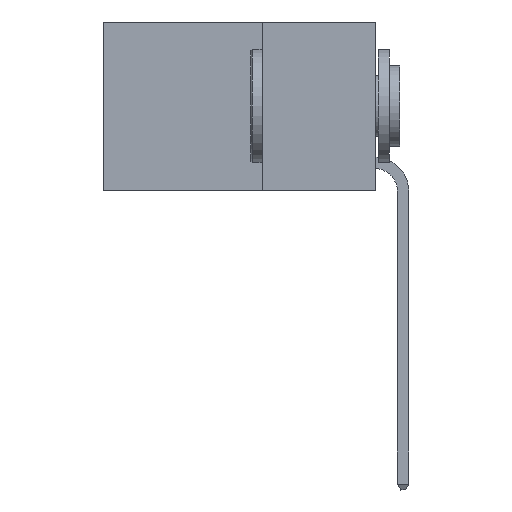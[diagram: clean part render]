
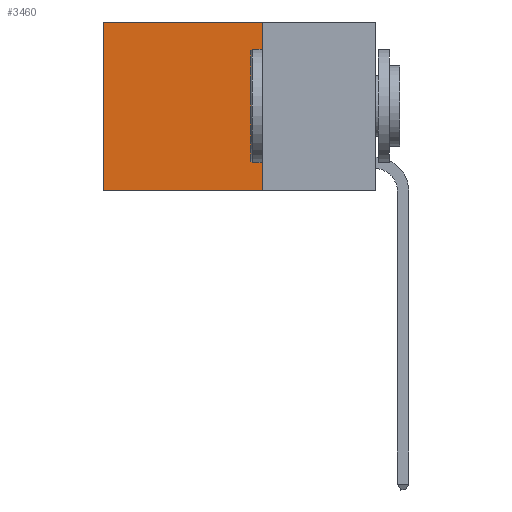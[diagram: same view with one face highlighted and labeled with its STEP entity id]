
A CAD part, left-side view. The second image highlights one B-rep face of the part: STEP entity #3460.
In plain terms, the highlighted planar face has unit normal (-1, 0, 0).
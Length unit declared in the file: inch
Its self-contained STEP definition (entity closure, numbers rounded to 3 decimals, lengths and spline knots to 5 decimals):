
#1109 = VERTEX_POINT ( 'NONE', #20126 ) ;
#1355 = ORIENTED_EDGE ( 'NONE', *, *, #22848, .T. ) ;
#1933 = CARTESIAN_POINT ( 'NONE',  ( 0.2625, 0.25, 0. ) ) ;
#2531 = DIRECTION ( 'NONE',  ( 1., 0., 0. ) ) ;
#3460 = ADVANCED_FACE ( 'NONE', ( #25578 ), #28165, .F. ) ;
#7009 = CARTESIAN_POINT ( 'NONE',  ( 0.2625, 0.6, 0. ) ) ;
#8017 = LINE ( 'NONE', #26478, #14754 ) ;
#8722 = EDGE_CURVE ( 'NONE', #28034, #11295, #30033, .T. ) ;
#8973 = DIRECTION ( 'NONE',  ( 0., 0., -1. ) ) ;
#8996 = CARTESIAN_POINT ( 'NONE',  ( 0.2625, 0.6, 0. ) ) ;
#9184 = VERTEX_POINT ( 'NONE', #20708 ) ;
#10628 = EDGE_CURVE ( 'NONE', #9184, #1109, #20876, .T. ) ;
#11295 = VERTEX_POINT ( 'NONE', #19718 ) ;
#14113 = ORIENTED_EDGE ( 'NONE', *, *, #15161, .F. ) ;
#14172 = VECTOR ( 'NONE', #27243, 39.37008 ) ;
#14754 = VECTOR ( 'NONE', #16878, 39.37008 ) ;
#15161 = EDGE_CURVE ( 'NONE', #1109, #11295, #8017, .T. ) ;
#15800 = AXIS2_PLACEMENT_3D ( 'NONE', #18413, #2531, #30142 ) ;
#16878 = DIRECTION ( 'NONE',  ( 0., 1., 0. ) ) ;
#17940 = CARTESIAN_POINT ( 'NONE',  ( 0.2625, 0.25, 0. ) ) ;
#18413 = CARTESIAN_POINT ( 'NONE',  ( 0.2625, 0.25, 0. ) ) ;
#18450 = DIRECTION ( 'NONE',  ( 0., 0., -1. ) ) ;
#18887 = ORIENTED_EDGE ( 'NONE', *, *, #10628, .F. ) ;
#19718 = CARTESIAN_POINT ( 'NONE',  ( 0.2625, 0.6, -0.37 ) ) ;
#19976 = VECTOR ( 'NONE', #8973, 39.37008 ) ;
#20126 = CARTESIAN_POINT ( 'NONE',  ( 0.2625, 0.25, -0.37 ) ) ;
#20234 = LINE ( 'NONE', #17940, #14172 ) ;
#20385 = EDGE_LOOP ( 'NONE', ( #25705, #14113, #18887, #1355 ) ) ;
#20708 = CARTESIAN_POINT ( 'NONE',  ( 0.2625, 0.25, 0. ) ) ;
#20876 = LINE ( 'NONE', #1933, #19976 ) ;
#22848 = EDGE_CURVE ( 'NONE', #9184, #28034, #20234, .T. ) ;
#25263 = VECTOR ( 'NONE', #18450, 39.37008 ) ;
#25578 = FACE_OUTER_BOUND ( 'NONE', #20385, .T. ) ;
#25705 = ORIENTED_EDGE ( 'NONE', *, *, #8722, .T. ) ;
#26478 = CARTESIAN_POINT ( 'NONE',  ( 0.2625, 0.25, -0.37 ) ) ;
#27243 = DIRECTION ( 'NONE',  ( 0., 1., 0. ) ) ;
#28034 = VERTEX_POINT ( 'NONE', #7009 ) ;
#28165 = PLANE ( 'NONE',  #15800 ) ;
#30033 = LINE ( 'NONE', #8996, #25263 ) ;
#30142 = DIRECTION ( 'NONE',  ( 0., 0., -1. ) ) ;
